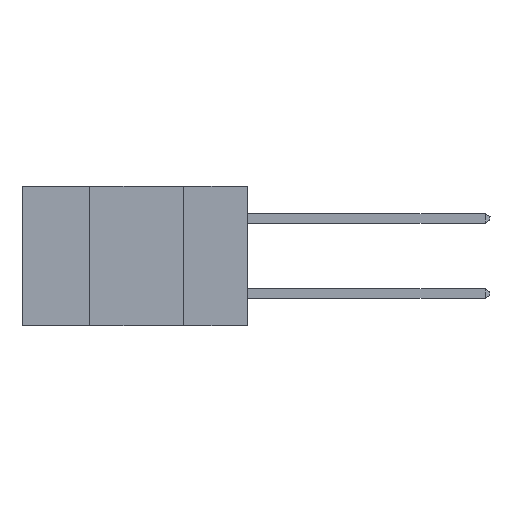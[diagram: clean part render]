
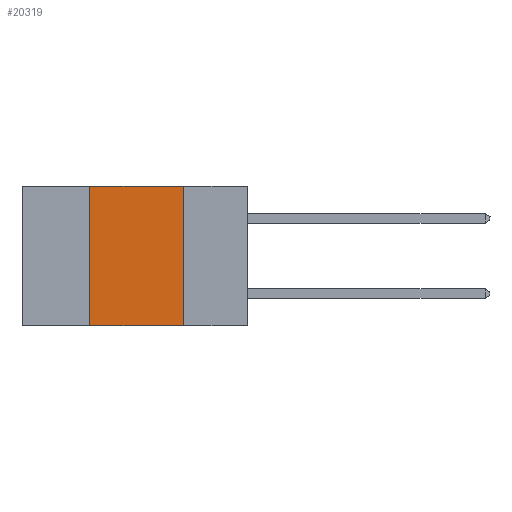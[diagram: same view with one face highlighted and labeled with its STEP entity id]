
A CAD part, left-side view. The second image highlights one B-rep face of the part: STEP entity #20319.
In plain terms, the highlighted planar face has unit normal (-1, 0, 0).
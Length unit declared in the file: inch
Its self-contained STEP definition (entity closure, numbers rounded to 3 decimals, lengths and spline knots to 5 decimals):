
#750 = ORIENTED_EDGE ( 'NONE', *, *, #3192, .T. ) ;
#1010 = ORIENTED_EDGE ( 'NONE', *, *, #14619, .F. ) ;
#1546 = LINE ( 'NONE', #7616, #7136 ) ;
#1765 = CARTESIAN_POINT ( 'NONE',  ( 0., 0.42, 0. ) ) ;
#1978 = CARTESIAN_POINT ( 'NONE',  ( 0., 0.42, -0.37 ) ) ;
#2315 = CARTESIAN_POINT ( 'NONE',  ( 0., 0.6, 0. ) ) ;
#2410 = LINE ( 'NONE', #19709, #6200 ) ;
#3192 = EDGE_CURVE ( 'NONE', #10007, #11686, #2410, .T. ) ;
#5177 = CARTESIAN_POINT ( 'NONE',  ( 0., 0.42, -0.37 ) ) ;
#5184 = ORIENTED_EDGE ( 'NONE', *, *, #9612, .F. ) ;
#6200 = VECTOR ( 'NONE', #10255, 39.37008 ) ;
#6248 = DIRECTION ( 'NONE',  ( 0., 0., -1. ) ) ;
#6319 = CARTESIAN_POINT ( 'NONE',  ( 0., 0.17, -0.37 ) ) ;
#7136 = VECTOR ( 'NONE', #6248, 39.37008 ) ;
#7616 = CARTESIAN_POINT ( 'NONE',  ( 0., 0.17, -0.37 ) ) ;
#9202 = PLANE ( 'NONE',  #16342 ) ;
#9266 = EDGE_CURVE ( 'NONE', #17770, #11844, #10469, .T. ) ;
#9612 = EDGE_CURVE ( 'NONE', #10007, #17770, #16225, .T. ) ;
#9973 = CARTESIAN_POINT ( 'NONE',  ( 0., 0.17, 0. ) ) ;
#10007 = VERTEX_POINT ( 'NONE', #5177 ) ;
#10255 = DIRECTION ( 'NONE',  ( 0., -1., 0. ) ) ;
#10468 = FACE_OUTER_BOUND ( 'NONE', #20229, .T. ) ;
#10469 = LINE ( 'NONE', #2315, #12681 ) ;
#10779 = CARTESIAN_POINT ( 'NONE',  ( 0., 0.6, 0. ) ) ;
#11393 = DIRECTION ( 'NONE',  ( 0., 0., 1. ) ) ;
#11686 = VERTEX_POINT ( 'NONE', #6319 ) ;
#11844 = VERTEX_POINT ( 'NONE', #9973 ) ;
#12681 = VECTOR ( 'NONE', #13613, 39.37008 ) ;
#13613 = DIRECTION ( 'NONE',  ( 0., -1., 0. ) ) ;
#13918 = DIRECTION ( 'NONE',  ( 1., 0., 0. ) ) ;
#14619 = EDGE_CURVE ( 'NONE', #11844, #11686, #1546, .T. ) ;
#15377 = VECTOR ( 'NONE', #11393, 39.37008 ) ;
#15555 = ORIENTED_EDGE ( 'NONE', *, *, #9266, .F. ) ;
#16225 = LINE ( 'NONE', #1978, #15377 ) ;
#16342 = AXIS2_PLACEMENT_3D ( 'NONE', #10779, #13918, #20021 ) ;
#17770 = VERTEX_POINT ( 'NONE', #1765 ) ;
#19709 = CARTESIAN_POINT ( 'NONE',  ( 0., 0.6, -0.37 ) ) ;
#20021 = DIRECTION ( 'NONE',  ( 0., 0., -1. ) ) ;
#20229 = EDGE_LOOP ( 'NONE', ( #1010, #15555, #5184, #750 ) ) ;
#20319 = ADVANCED_FACE ( 'NONE', ( #10468 ), #9202, .F. ) ;
